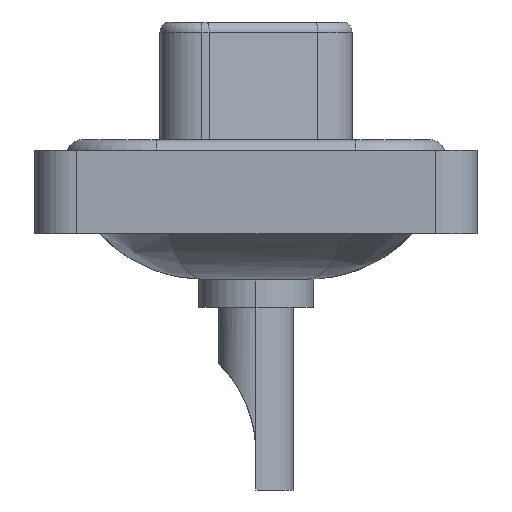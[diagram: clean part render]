
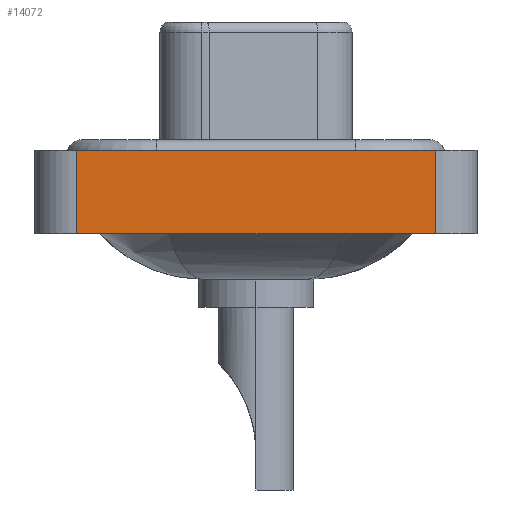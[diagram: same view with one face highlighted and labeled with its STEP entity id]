
A CAD part, left-side view. The second image highlights one B-rep face of the part: STEP entity #14072.
In plain terms, the highlighted planar face has unit normal (-1, 0, 0).
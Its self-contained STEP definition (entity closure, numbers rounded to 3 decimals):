
#220 = CARTESIAN_POINT ( 'NONE',  ( -7.3, -8.55, 0.4 ) ) ;
#423 = CARTESIAN_POINT ( 'NONE',  ( -7.3, 8.55, 0.4 ) ) ;
#1369 = EDGE_CURVE ( 'NONE', #7337, #3436, #8701, .T. ) ;
#1580 = PLANE ( 'NONE',  #14814 ) ;
#1667 = CARTESIAN_POINT ( 'NONE',  ( -7.3, -8.55, -3.6 ) ) ;
#2011 = VERTEX_POINT ( 'NONE', #220 ) ;
#2911 = ORIENTED_EDGE ( 'NONE', *, *, #12590, .F. ) ;
#3436 = VERTEX_POINT ( 'NONE', #423 ) ;
#4023 = VECTOR ( 'NONE', #6391, 1000. ) ;
#4193 = FACE_OUTER_BOUND ( 'NONE', #12963, .T. ) ;
#5024 = CARTESIAN_POINT ( 'NONE',  ( -7.3, -8.55, 0.4 ) ) ;
#5103 = CARTESIAN_POINT ( 'NONE',  ( -7.3, 8.55, -3.6 ) ) ;
#5794 = LINE ( 'NONE', #13219, #6269 ) ;
#6248 = CARTESIAN_POINT ( 'NONE',  ( -7.3, 8.55, -3.6 ) ) ;
#6269 = VECTOR ( 'NONE', #12217, 1000. ) ;
#6391 = DIRECTION ( 'NONE',  ( 0., -1., 0. ) ) ;
#7069 = VERTEX_POINT ( 'NONE', #9669 ) ;
#7337 = VERTEX_POINT ( 'NONE', #6248 ) ;
#7660 = EDGE_CURVE ( 'NONE', #7337, #7069, #5794, .T. ) ;
#8217 = EDGE_CURVE ( 'NONE', #7069, #2011, #13943, .T. ) ;
#8701 = LINE ( 'NONE', #5103, #13559 ) ;
#9047 = ORIENTED_EDGE ( 'NONE', *, *, #7660, .T. ) ;
#9368 = DIRECTION ( 'NONE',  ( -1., 0., 0. ) ) ;
#9669 = CARTESIAN_POINT ( 'NONE',  ( -7.3, -8.55, -3.6 ) ) ;
#10149 = ORIENTED_EDGE ( 'NONE', *, *, #8217, .T. ) ;
#10292 = DIRECTION ( 'NONE',  ( 0., 0., 1. ) ) ;
#11379 = LINE ( 'NONE', #5024, #4023 ) ;
#12201 = VECTOR ( 'NONE', #13641, 1000. ) ;
#12217 = DIRECTION ( 'NONE',  ( 0., -1., 0. ) ) ;
#12590 = EDGE_CURVE ( 'NONE', #3436, #2011, #11379, .T. ) ;
#12963 = EDGE_LOOP ( 'NONE', ( #10149, #2911, #14199, #9047 ) ) ;
#13219 = CARTESIAN_POINT ( 'NONE',  ( -7.3, -8.55, -3.6 ) ) ;
#13559 = VECTOR ( 'NONE', #10292, 1000. ) ;
#13641 = DIRECTION ( 'NONE',  ( 0., 0., 1. ) ) ;
#13943 = LINE ( 'NONE', #15199, #12201 ) ;
#14072 = ADVANCED_FACE ( 'NONE', ( #4193 ), #1580, .T. ) ;
#14199 = ORIENTED_EDGE ( 'NONE', *, *, #1369, .F. ) ;
#14304 = DIRECTION ( 'NONE',  ( 0., 0., 1. ) ) ;
#14814 = AXIS2_PLACEMENT_3D ( 'NONE', #1667, #9368, #14304 ) ;
#15199 = CARTESIAN_POINT ( 'NONE',  ( -7.3, -8.55, -3.6 ) ) ;
